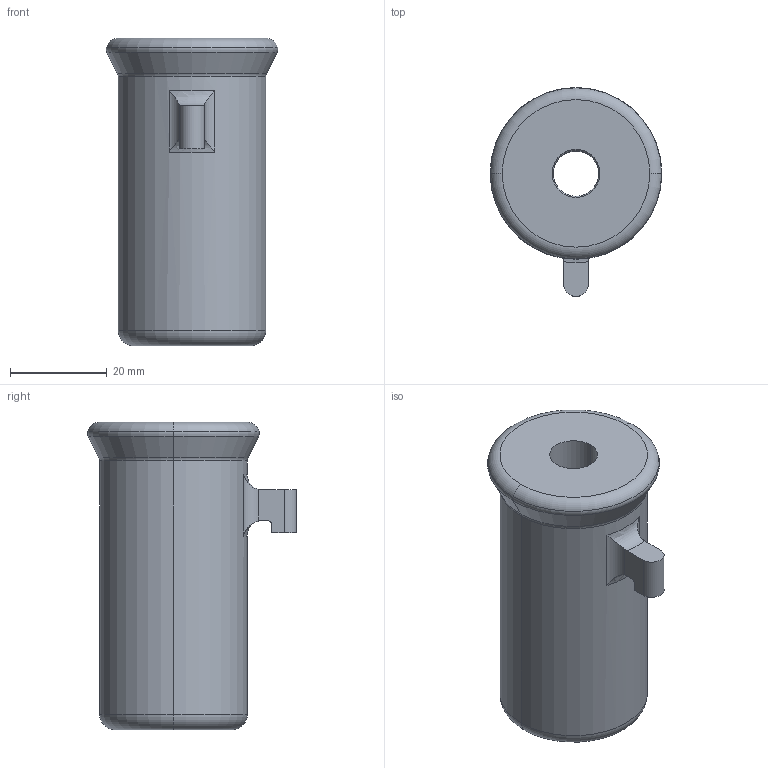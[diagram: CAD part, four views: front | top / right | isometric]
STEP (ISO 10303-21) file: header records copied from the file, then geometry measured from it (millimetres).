
FILE_DESCRIPTION (( 'STEP AP214' ), '1' );
FILE_NAME ('380 barrel (threaded).STEP', '2013-05-27T22:45:49', ( 'Asher' ), ( '' ), 'SwSTEP 2.0', 'SolidWorks 2013', '' );
FILE_SCHEMA (( 'AUTOMOTIVE_DESIGN' ));
Length unit declared in the file: millimetre
Products named in the file (1): 380 barrel (threaded)
Bounding box: 35.48 x 43.14 x 63.5 mm (x, y, z)
Volume: 43085.6 mm3; surface area: 9649.5 mm2
Topology: 1 solids, 1 shells, 52 faces, 132 edges, 83 vertices
Faces by surface type: plane 23, torus 16, cylinder 11, cone 2
Entity records: 1709 total; most frequent: CARTESIAN_POINT 414, DIRECTION 271, ORIENTED_EDGE 264, EDGE_CURVE 132, AXIS2_PLACEMENT_3D 110, VERTEX_POINT 83, CIRCLE 57, EDGE_LOOP 55
